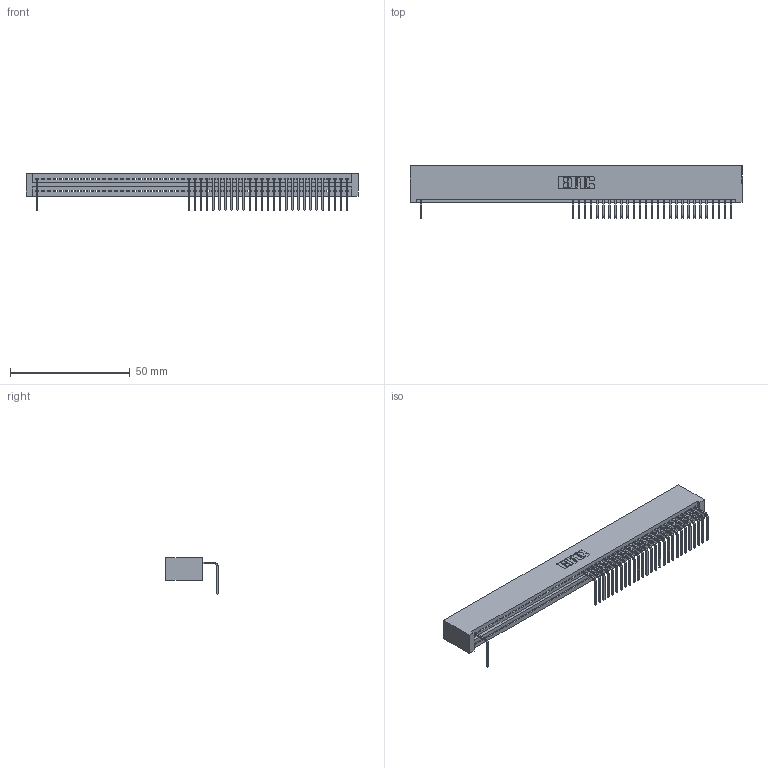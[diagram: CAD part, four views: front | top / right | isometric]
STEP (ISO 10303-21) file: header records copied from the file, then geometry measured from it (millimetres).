
FILE_DESCRIPTION (( 'STEP AP203' ), '1' );
FILE_NAME ('345-052-558-101.STEP', '2018-09-23T00:06:02', ( '' ), ( '' ), 'SwSTEP 2.0', 'SolidWorks 2016', '' );
FILE_SCHEMA (( 'CONFIG_CONTROL_DESIGN' ));
Length unit declared in the file: inch
Products named in the file (3): 345 Part_No Mounting Lugs; 345-292-001_558 Tail - 2; 345-052-558-101
Assembly tree (29 placements, depth 2):
  345-052-558-101
    345 Part_No Mounting Lugs
    345-292-001_558 Tail - 2  x28
Bounding box: 138.68 x 21.83 x 15.37 mm (x, y, z)
Volume: 13657.1 mm3; surface area: 17563.8 mm2
Topology: 29 solids, 29 shells, 2182 faces, 6709 edges, 4434 vertices
Faces by surface type: plane 1588, cylinder 594
Entity records: 36829 total; most frequent: ORIENTED_EDGE 6506, CARTESIAN_POINT 6496, DIRECTION 5625, EDGE_CURVE 3253, VECTOR 2921, LINE 2921, VERTEX_POINT 2166, AXIS2_PLACEMENT_3D 1352
